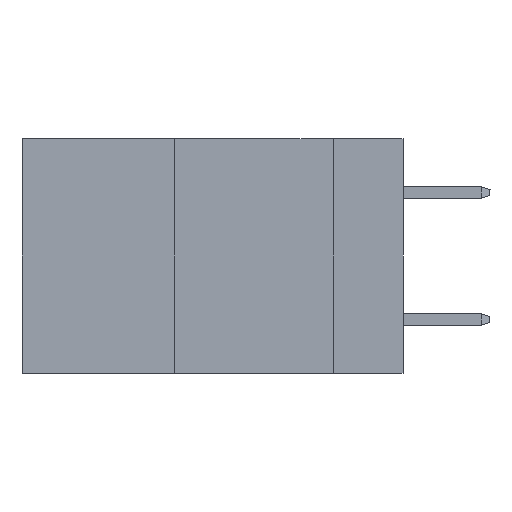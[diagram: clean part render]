
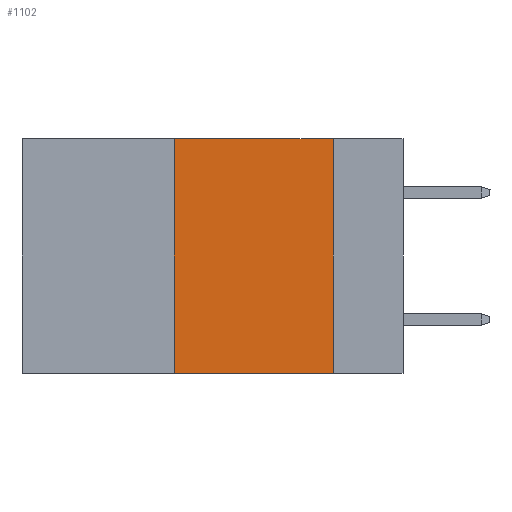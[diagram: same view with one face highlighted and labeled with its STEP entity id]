
A CAD part, left-side view. The second image highlights one B-rep face of the part: STEP entity #1102.
In plain terms, the highlighted planar face has unit normal (-1, 0, 0).
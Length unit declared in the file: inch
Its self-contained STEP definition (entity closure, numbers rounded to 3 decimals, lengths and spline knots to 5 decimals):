
#279 = ORIENTED_EDGE ( 'NONE', *, *, #12271, .T. ) ;
#1102 = ADVANCED_FACE ( 'NONE', ( #23284 ), #15610, .F. ) ;
#1145 = DIRECTION ( 'NONE',  ( 0., 0., -1. ) ) ;
#1856 = EDGE_CURVE ( 'NONE', #9650, #30903, #33683, .T. ) ;
#2489 = EDGE_CURVE ( 'NONE', #16065, #9650, #29537, .T. ) ;
#4837 = CARTESIAN_POINT ( 'NONE',  ( 0., 0.36, -0.37 ) ) ;
#9650 = VERTEX_POINT ( 'NONE', #11474 ) ;
#9992 = CARTESIAN_POINT ( 'NONE',  ( 0., 0.11, -0.37 ) ) ;
#11474 = CARTESIAN_POINT ( 'NONE',  ( 0., 0.11, 0. ) ) ;
#12271 = EDGE_CURVE ( 'NONE', #25830, #30903, #29354, .T. ) ;
#13488 = DIRECTION ( 'NONE',  ( 0., -1., 0. ) ) ;
#14258 = ORIENTED_EDGE ( 'NONE', *, *, #2489, .F. ) ;
#15267 = DIRECTION ( 'NONE',  ( 0., -1., 0. ) ) ;
#15610 = PLANE ( 'NONE',  #27391 ) ;
#15800 = DIRECTION ( 'NONE',  ( 1., 0., 0. ) ) ;
#15980 = VECTOR ( 'NONE', #1145, 39.37008 ) ;
#16065 = VERTEX_POINT ( 'NONE', #20493 ) ;
#16733 = EDGE_CURVE ( 'NONE', #25830, #16065, #20989, .T. ) ;
#18169 = VECTOR ( 'NONE', #31876, 39.37008 ) ;
#18312 = CARTESIAN_POINT ( 'NONE',  ( 0., 0.36, 0. ) ) ;
#19179 = CARTESIAN_POINT ( 'NONE',  ( 0., 0.6, 0. ) ) ;
#19630 = VECTOR ( 'NONE', #13488, 39.37008 ) ;
#20253 = VECTOR ( 'NONE', #15267, 39.37008 ) ;
#20493 = CARTESIAN_POINT ( 'NONE',  ( 0., 0.36, 0. ) ) ;
#20989 = LINE ( 'NONE', #18312, #18169 ) ;
#21343 = ORIENTED_EDGE ( 'NONE', *, *, #1856, .F. ) ;
#21512 = CARTESIAN_POINT ( 'NONE',  ( 0., 0.6, -0.37 ) ) ;
#23282 = EDGE_LOOP ( 'NONE', ( #21343, #14258, #31265, #279 ) ) ;
#23284 = FACE_OUTER_BOUND ( 'NONE', #23282, .T. ) ;
#23637 = DIRECTION ( 'NONE',  ( 0., 0., -1. ) ) ;
#25830 = VERTEX_POINT ( 'NONE', #4837 ) ;
#26012 = CARTESIAN_POINT ( 'NONE',  ( 0., 0.11, 0. ) ) ;
#27391 = AXIS2_PLACEMENT_3D ( 'NONE', #31475, #15800, #23637 ) ;
#29354 = LINE ( 'NONE', #21512, #20253 ) ;
#29537 = LINE ( 'NONE', #19179, #19630 ) ;
#30903 = VERTEX_POINT ( 'NONE', #9992 ) ;
#31265 = ORIENTED_EDGE ( 'NONE', *, *, #16733, .F. ) ;
#31475 = CARTESIAN_POINT ( 'NONE',  ( 0., 0.6, 0. ) ) ;
#31876 = DIRECTION ( 'NONE',  ( 0., 0., 1. ) ) ;
#33683 = LINE ( 'NONE', #26012, #15980 ) ;
